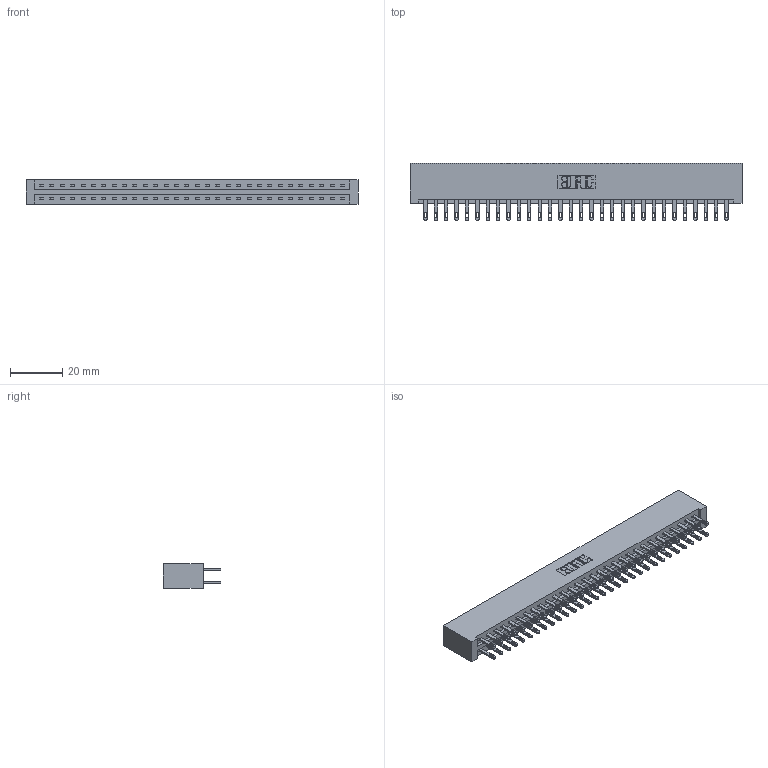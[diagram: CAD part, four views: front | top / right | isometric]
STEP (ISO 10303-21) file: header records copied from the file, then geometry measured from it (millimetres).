
FILE_DESCRIPTION (( 'STEP AP203' ), '1' );
FILE_NAME ('337-060-500-201.STEP', '2018-08-10T06:47:32', ( '' ), ( '' ), 'SwSTEP 2.0', 'SolidWorks 2016', '' );
FILE_SCHEMA (( 'CONFIG_CONTROL_DESIGN' ));
Length unit declared in the file: inch
Products named in the file (3): 337 Part_No Mounting Lugs; 345-292-001_345-293-100; 337-060-500-201
Assembly tree (61 placements, depth 2):
  337-060-500-201
    337 Part_No Mounting Lugs
    345-292-001_345-293-100  x60
Bounding box: 126.75 x 21.85 x 9.4 mm (x, y, z)
Volume: 14141.9 mm3; surface area: 16592.7 mm2
Topology: 61 solids, 61 shells, 3106 faces, 9467 edges, 6310 vertices
Faces by surface type: plane 1986, cylinder 1120
Entity records: 24465 total; most frequent: CARTESIAN_POINT 4130, ORIENTED_EDGE 4066, DIRECTION 3529, EDGE_CURVE 2033, LINE 1909, VECTOR 1909, VERTEX_POINT 1354, AXIS2_PLACEMENT_3D 810
